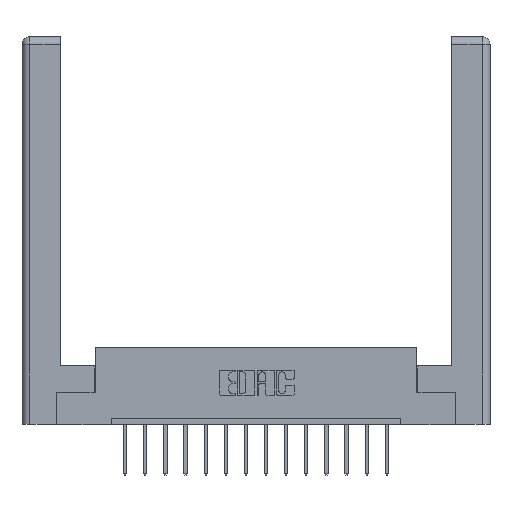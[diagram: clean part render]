
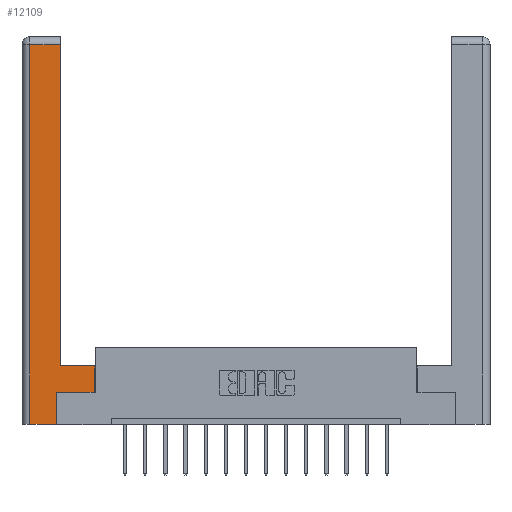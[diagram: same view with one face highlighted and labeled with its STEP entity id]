
A CAD part, top view. The second image highlights one B-rep face of the part: STEP entity #12109.
In plain terms, the highlighted planar face has unit normal (0, 0, 1).
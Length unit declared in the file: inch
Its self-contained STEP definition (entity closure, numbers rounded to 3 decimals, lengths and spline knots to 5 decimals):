
#138 = EDGE_CURVE ( 'NONE', #10081, #7410, #11565, .T. ) ;
#289 = LINE ( 'NONE', #8843, #10787 ) ;
#430 = VERTEX_POINT ( 'NONE', #9758 ) ;
#634 = CARTESIAN_POINT ( 'NONE',  ( 0.265, 0., 0. ) ) ;
#1242 = VERTEX_POINT ( 'NONE', #6533 ) ;
#1471 = DIRECTION ( 'NONE',  ( 0., 0., -1. ) ) ;
#1649 = EDGE_CURVE ( 'NONE', #430, #11636, #7607, .T. ) ;
#2240 = ORIENTED_EDGE ( 'NONE', *, *, #3002, .T. ) ;
#2270 = DIRECTION ( 'NONE',  ( 0., 1., 0. ) ) ;
#2748 = CARTESIAN_POINT ( 'NONE',  ( 0.565, 0.245, 0. ) ) ;
#3002 = EDGE_CURVE ( 'NONE', #11636, #6253, #289, .T. ) ;
#3091 = LINE ( 'NONE', #11463, #5720 ) ;
#3286 = CARTESIAN_POINT ( 'NONE',  ( 0.295, 0.45, 0. ) ) ;
#3391 = LINE ( 'NONE', #11392, #3823 ) ;
#3823 = VECTOR ( 'NONE', #6136, 39.37008 ) ;
#4058 = VECTOR ( 'NONE', #6396, 39.37008 ) ;
#4163 = EDGE_CURVE ( 'NONE', #6844, #10081, #3091, .T. ) ;
#4340 = CARTESIAN_POINT ( 'NONE',  ( 0.265, 0., 0. ) ) ;
#4542 = CARTESIAN_POINT ( 'NONE',  ( 0.265, 0.245, 0. ) ) ;
#4676 = LINE ( 'NONE', #7090, #13726 ) ;
#4835 = EDGE_CURVE ( 'NONE', #1242, #10466, #4676, .T. ) ;
#5371 = DIRECTION ( 'NONE',  ( -1., 0., 0. ) ) ;
#5720 = VECTOR ( 'NONE', #2270, 39.37008 ) ;
#5756 = CARTESIAN_POINT ( 'NONE',  ( 0.0615, 2.94, 0. ) ) ;
#5841 = VECTOR ( 'NONE', #12920, 39.37008 ) ;
#6136 = DIRECTION ( 'NONE',  ( -1., 0., 0. ) ) ;
#6253 = VERTEX_POINT ( 'NONE', #4542 ) ;
#6396 = DIRECTION ( 'NONE',  ( 1., 0., 0. ) ) ;
#6533 = CARTESIAN_POINT ( 'NONE',  ( 0.565, 0.245, 0. ) ) ;
#6844 = VERTEX_POINT ( 'NONE', #3286 ) ;
#7090 = CARTESIAN_POINT ( 'NONE',  ( 0.565, 0.45, 0. ) ) ;
#7410 = VERTEX_POINT ( 'NONE', #5756 ) ;
#7607 = LINE ( 'NONE', #4340, #11043 ) ;
#7966 = FACE_OUTER_BOUND ( 'NONE', #8835, .T. ) ;
#8835 = EDGE_LOOP ( 'NONE', ( #8884, #11443, #16471, #9871, #2240, #9033, #11923, #15671 ) ) ;
#8843 = CARTESIAN_POINT ( 'NONE',  ( 0.265, 0.245, 0. ) ) ;
#8884 = ORIENTED_EDGE ( 'NONE', *, *, #4163, .T. ) ;
#8905 = EDGE_CURVE ( 'NONE', #7410, #430, #9679, .T. ) ;
#9033 = ORIENTED_EDGE ( 'NONE', *, *, #13208, .T. ) ;
#9349 = VECTOR ( 'NONE', #5371, 39.37008 ) ;
#9372 = CARTESIAN_POINT ( 'NONE',  ( 0.0615, 2.94, 0. ) ) ;
#9374 = EDGE_CURVE ( 'NONE', #10466, #6844, #3391, .T. ) ;
#9679 = LINE ( 'NONE', #13138, #5841 ) ;
#9699 = LINE ( 'NONE', #2748, #4058 ) ;
#9758 = CARTESIAN_POINT ( 'NONE',  ( 0.0615, 0., 0. ) ) ;
#9871 = ORIENTED_EDGE ( 'NONE', *, *, #1649, .T. ) ;
#10081 = VERTEX_POINT ( 'NONE', #14255 ) ;
#10252 = DIRECTION ( 'NONE',  ( 0., 1., 0. ) ) ;
#10458 = DIRECTION ( 'NONE',  ( -1., 0., 0. ) ) ;
#10466 = VERTEX_POINT ( 'NONE', #12699 ) ;
#10787 = VECTOR ( 'NONE', #10252, 39.37008 ) ;
#11043 = VECTOR ( 'NONE', #12373, 39.37008 ) ;
#11392 = CARTESIAN_POINT ( 'NONE',  ( 0.295, 0.45, 0. ) ) ;
#11443 = ORIENTED_EDGE ( 'NONE', *, *, #138, .T. ) ;
#11463 = CARTESIAN_POINT ( 'NONE',  ( 0.295, 3., 0. ) ) ;
#11565 = LINE ( 'NONE', #9372, #9349 ) ;
#11636 = VERTEX_POINT ( 'NONE', #634 ) ;
#11923 = ORIENTED_EDGE ( 'NONE', *, *, #4835, .T. ) ;
#12109 = ADVANCED_FACE ( 'NONE', ( #7966 ), #15640, .F. ) ;
#12373 = DIRECTION ( 'NONE',  ( 1., 0., 0. ) ) ;
#12418 = DIRECTION ( 'NONE',  ( 0., 1., 0. ) ) ;
#12699 = CARTESIAN_POINT ( 'NONE',  ( 0.565, 0.45, 0. ) ) ;
#12920 = DIRECTION ( 'NONE',  ( 0., -1., 0. ) ) ;
#13016 = CARTESIAN_POINT ( 'NONE',  ( 0., 0., 0. ) ) ;
#13138 = CARTESIAN_POINT ( 'NONE',  ( 0.0615, 0., 0. ) ) ;
#13208 = EDGE_CURVE ( 'NONE', #6253, #1242, #9699, .T. ) ;
#13726 = VECTOR ( 'NONE', #12418, 39.37008 ) ;
#14255 = CARTESIAN_POINT ( 'NONE',  ( 0.295, 2.94, 0. ) ) ;
#15127 = AXIS2_PLACEMENT_3D ( 'NONE', #13016, #1471, #10458 ) ;
#15640 = PLANE ( 'NONE',  #15127 ) ;
#15671 = ORIENTED_EDGE ( 'NONE', *, *, #9374, .T. ) ;
#16471 = ORIENTED_EDGE ( 'NONE', *, *, #8905, .T. ) ;
